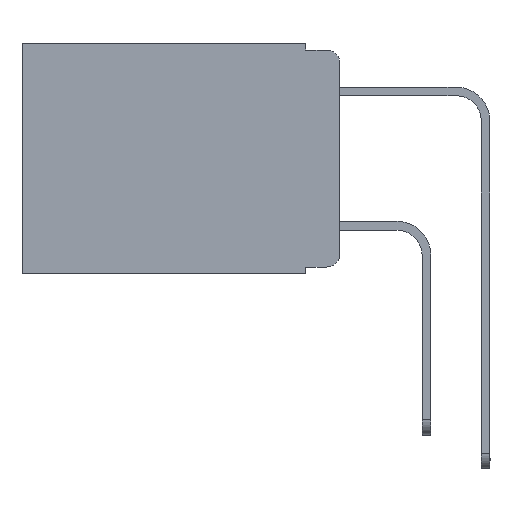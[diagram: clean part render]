
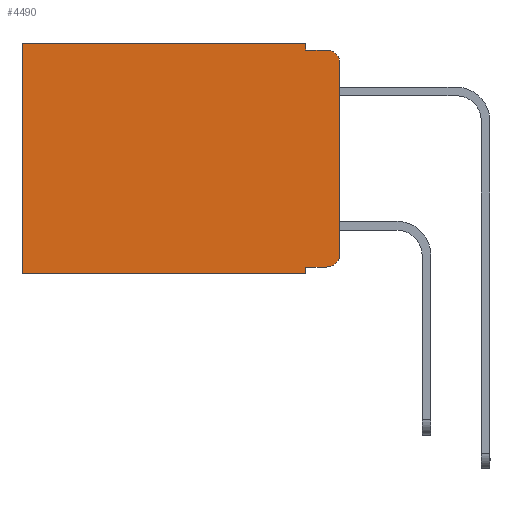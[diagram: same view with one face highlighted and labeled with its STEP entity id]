
A CAD part, left-side view. The second image highlights one B-rep face of the part: STEP entity #4490.
In plain terms, the highlighted planar face has unit normal (-1, 0, 0).
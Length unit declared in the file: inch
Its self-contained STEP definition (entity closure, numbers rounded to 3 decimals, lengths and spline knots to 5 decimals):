
#437 = VERTEX_POINT ( 'NONE', #2041 ) ;
#728 = VERTEX_POINT ( 'NONE', #4358 ) ;
#763 = CARTESIAN_POINT ( 'NONE',  ( 0.298, 0.473, 0. ) ) ;
#826 = CIRCLE ( 'NONE', #8982, 0.02 ) ;
#921 = LINE ( 'NONE', #9403, #10901 ) ;
#1090 = EDGE_CURVE ( 'NONE', #4123, #8943, #9931, .T. ) ;
#1230 = DIRECTION ( 'NONE',  ( 0., 0., -1. ) ) ;
#1299 = LINE ( 'NONE', #10567, #8988 ) ;
#1329 = LINE ( 'NONE', #4729, #8446 ) ;
#1364 = VECTOR ( 'NONE', #8169, 39.37008 ) ;
#1479 = LINE ( 'NONE', #5713, #7420 ) ;
#1559 = DIRECTION ( 'NONE',  ( -1., 0., 0. ) ) ;
#1615 = ORIENTED_EDGE ( 'NONE', *, *, #9752, .F. ) ;
#1961 = LINE ( 'NONE', #5349, #1364 ) ;
#2041 = CARTESIAN_POINT ( 'NONE',  ( 0.298, 0.051, -0.01 ) ) ;
#2254 = CARTESIAN_POINT ( 'NONE',  ( 0.298, 0., -0.313 ) ) ;
#2288 = ORIENTED_EDGE ( 'NONE', *, *, #4463, .F. ) ;
#2377 = DIRECTION ( 'NONE',  ( 0., 0., -1. ) ) ;
#2452 = ORIENTED_EDGE ( 'NONE', *, *, #4961, .T. ) ;
#2456 = CARTESIAN_POINT ( 'NONE',  ( 0.298, 0., 0. ) ) ;
#2499 = CARTESIAN_POINT ( 'NONE',  ( 0.298, 0.02, -0.333 ) ) ;
#2917 = VERTEX_POINT ( 'NONE', #2254 ) ;
#2952 = AXIS2_PLACEMENT_3D ( 'NONE', #7912, #4640, #5576 ) ;
#2970 = VECTOR ( 'NONE', #5854, 39.37008 ) ;
#3091 = DIRECTION ( 'NONE',  ( 0., 0., -1. ) ) ;
#3150 = ORIENTED_EDGE ( 'NONE', *, *, #9000, .F. ) ;
#3417 = CARTESIAN_POINT ( 'NONE',  ( 0.298, 0.051, 0. ) ) ;
#3460 = ORIENTED_EDGE ( 'NONE', *, *, #1090, .T. ) ;
#4003 = CARTESIAN_POINT ( 'NONE',  ( 0.298, 0.02, -0.03 ) ) ;
#4123 = VERTEX_POINT ( 'NONE', #763 ) ;
#4358 = CARTESIAN_POINT ( 'NONE',  ( 0.298, 0., -0.03 ) ) ;
#4463 = EDGE_CURVE ( 'NONE', #437, #10310, #4692, .T. ) ;
#4490 = ADVANCED_FACE ( 'NONE', ( #8967 ), #10472, .F. ) ;
#4640 = DIRECTION ( 'NONE',  ( 1., 0., 0. ) ) ;
#4688 = DIRECTION ( 'NONE',  ( 0., 0., -1. ) ) ;
#4692 = LINE ( 'NONE', #5528, #9693 ) ;
#4725 = VERTEX_POINT ( 'NONE', #7726 ) ;
#4729 = CARTESIAN_POINT ( 'NONE',  ( 0.298, 0.051, 0. ) ) ;
#4946 = EDGE_CURVE ( 'NONE', #5404, #4123, #1961, .T. ) ;
#4961 = EDGE_CURVE ( 'NONE', #10124, #2917, #5089, .T. ) ;
#5089 = CIRCLE ( 'NONE', #7926, 0.02 ) ;
#5349 = CARTESIAN_POINT ( 'NONE',  ( 0.298, 0., 0. ) ) ;
#5404 = VERTEX_POINT ( 'NONE', #3417 ) ;
#5528 = CARTESIAN_POINT ( 'NONE',  ( 0.298, 0.051, -0.01 ) ) ;
#5576 = DIRECTION ( 'NONE',  ( 0., 0., -1. ) ) ;
#5669 = EDGE_CURVE ( 'NONE', #9850, #8943, #1479, .T. ) ;
#5705 = EDGE_LOOP ( 'NONE', ( #1615, #6406, #2288, #8607, #7613, #3460, #7540, #3150, #9391, #2452 ) ) ;
#5713 = CARTESIAN_POINT ( 'NONE',  ( 0.298, 0., -0.343 ) ) ;
#5854 = DIRECTION ( 'NONE',  ( 0., 0., -1. ) ) ;
#5956 = LINE ( 'NONE', #2456, #2970 ) ;
#6121 = CARTESIAN_POINT ( 'NONE',  ( 0.298, 0.473, -0.343 ) ) ;
#6406 = ORIENTED_EDGE ( 'NONE', *, *, #8324, .T. ) ;
#6596 = CARTESIAN_POINT ( 'NONE',  ( 0.298, 0.473, 0. ) ) ;
#7420 = VECTOR ( 'NONE', #9927, 39.37008 ) ;
#7540 = ORIENTED_EDGE ( 'NONE', *, *, #5669, .F. ) ;
#7580 = EDGE_CURVE ( 'NONE', #4725, #10124, #921, .T. ) ;
#7613 = ORIENTED_EDGE ( 'NONE', *, *, #4946, .T. ) ;
#7726 = CARTESIAN_POINT ( 'NONE',  ( 0.298, 0.051, -0.333 ) ) ;
#7912 = CARTESIAN_POINT ( 'NONE',  ( 0.298, 0., 0. ) ) ;
#7926 = AXIS2_PLACEMENT_3D ( 'NONE', #10669, #8110, #1230 ) ;
#7977 = DIRECTION ( 'NONE',  ( 0., -1., 0. ) ) ;
#8110 = DIRECTION ( 'NONE',  ( -1., 0., 0. ) ) ;
#8169 = DIRECTION ( 'NONE',  ( 0., 1., 0. ) ) ;
#8324 = EDGE_CURVE ( 'NONE', #728, #10310, #826, .T. ) ;
#8334 = DIRECTION ( 'NONE',  ( 0., 0., -1. ) ) ;
#8341 = EDGE_CURVE ( 'NONE', #5404, #437, #1329, .T. ) ;
#8446 = VECTOR ( 'NONE', #8334, 39.37008 ) ;
#8510 = CARTESIAN_POINT ( 'NONE',  ( 0.298, 0.051, -0.343 ) ) ;
#8607 = ORIENTED_EDGE ( 'NONE', *, *, #8341, .F. ) ;
#8943 = VERTEX_POINT ( 'NONE', #6121 ) ;
#8967 = FACE_OUTER_BOUND ( 'NONE', #5705, .T. ) ;
#8982 = AXIS2_PLACEMENT_3D ( 'NONE', #4003, #1559, #2377 ) ;
#8988 = VECTOR ( 'NONE', #4688, 39.37008 ) ;
#9000 = EDGE_CURVE ( 'NONE', #4725, #9850, #1299, .T. ) ;
#9391 = ORIENTED_EDGE ( 'NONE', *, *, #7580, .T. ) ;
#9403 = CARTESIAN_POINT ( 'NONE',  ( 0.298, 0.051, -0.333 ) ) ;
#9693 = VECTOR ( 'NONE', #7977, 39.37008 ) ;
#9714 = CARTESIAN_POINT ( 'NONE',  ( 0.298, 0.02, -0.01 ) ) ;
#9752 = EDGE_CURVE ( 'NONE', #728, #2917, #5956, .T. ) ;
#9767 = VECTOR ( 'NONE', #3091, 39.37008 ) ;
#9850 = VERTEX_POINT ( 'NONE', #8510 ) ;
#9927 = DIRECTION ( 'NONE',  ( 0., 1., 0. ) ) ;
#9931 = LINE ( 'NONE', #6596, #9767 ) ;
#10124 = VERTEX_POINT ( 'NONE', #2499 ) ;
#10297 = DIRECTION ( 'NONE',  ( 0., -1., 0. ) ) ;
#10310 = VERTEX_POINT ( 'NONE', #9714 ) ;
#10472 = PLANE ( 'NONE',  #2952 ) ;
#10567 = CARTESIAN_POINT ( 'NONE',  ( 0.298, 0.051, 0. ) ) ;
#10669 = CARTESIAN_POINT ( 'NONE',  ( 0.298, 0.02, -0.313 ) ) ;
#10901 = VECTOR ( 'NONE', #10297, 39.37008 ) ;
